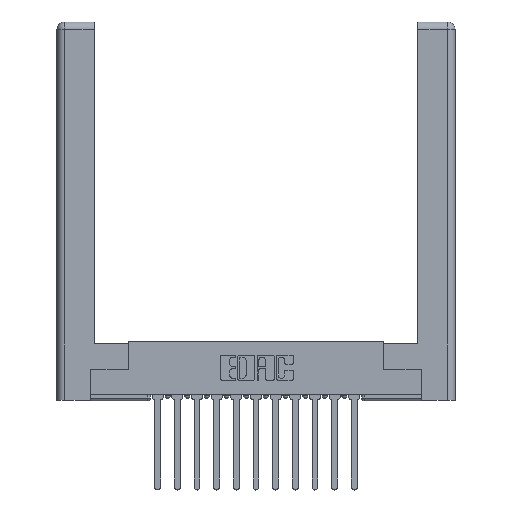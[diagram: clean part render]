
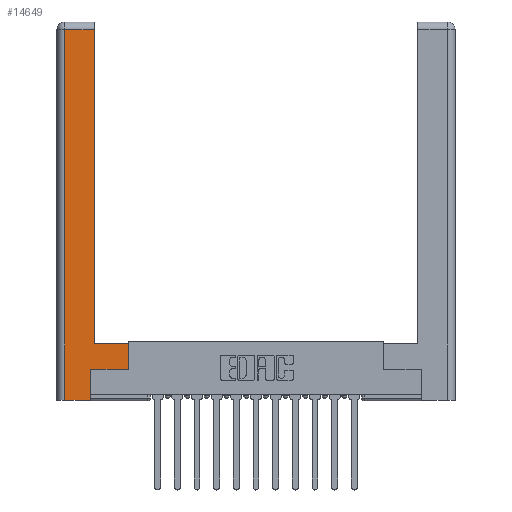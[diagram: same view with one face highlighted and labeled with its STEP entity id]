
A CAD part, top view. The second image highlights one B-rep face of the part: STEP entity #14649.
In plain terms, the highlighted planar face has unit normal (0, 0, 1).
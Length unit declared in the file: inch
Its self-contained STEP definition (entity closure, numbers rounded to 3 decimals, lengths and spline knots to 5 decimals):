
#219 = EDGE_CURVE ( 'NONE', #305, #6769, #8221, .T. ) ;
#305 = VERTEX_POINT ( 'NONE', #5192 ) ;
#957 = VERTEX_POINT ( 'NONE', #15986 ) ;
#1286 = DIRECTION ( 'NONE',  ( -1., 0., 0. ) ) ;
#1418 = DIRECTION ( 'NONE',  ( 0., 1., 0. ) ) ;
#1597 = CARTESIAN_POINT ( 'NONE',  ( 0.565, 0.45, 0. ) ) ;
#1611 = CARTESIAN_POINT ( 'NONE',  ( 0.565, 0.245, 0. ) ) ;
#1835 = VECTOR ( 'NONE', #6300, 39.37008 ) ;
#2227 = LINE ( 'NONE', #3310, #15348 ) ;
#2528 = VERTEX_POINT ( 'NONE', #7057 ) ;
#2570 = DIRECTION ( 'NONE',  ( 1., 0., 0. ) ) ;
#3310 = CARTESIAN_POINT ( 'NONE',  ( 0.265, 0.245, 0. ) ) ;
#3886 = CARTESIAN_POINT ( 'NONE',  ( 0.265, 0., 0. ) ) ;
#4019 = VECTOR ( 'NONE', #15083, 39.37008 ) ;
#4164 = EDGE_LOOP ( 'NONE', ( #5932, #5208, #7572, #6609, #14866, #4884, #8962, #14830 ) ) ;
#4169 = EDGE_CURVE ( 'NONE', #957, #11732, #12850, .T. ) ;
#4410 = LINE ( 'NONE', #11328, #4019 ) ;
#4884 = ORIENTED_EDGE ( 'NONE', *, *, #4169, .T. ) ;
#5192 = CARTESIAN_POINT ( 'NONE',  ( 0.0615, 0., 0. ) ) ;
#5208 = ORIENTED_EDGE ( 'NONE', *, *, #14543, .T. ) ;
#5555 = CARTESIAN_POINT ( 'NONE',  ( 0.0615, 2.94, 0. ) ) ;
#5618 = VECTOR ( 'NONE', #2570, 39.37008 ) ;
#5813 = DIRECTION ( 'NONE',  ( -1., 0., 0. ) ) ;
#5932 = ORIENTED_EDGE ( 'NONE', *, *, #9683, .T. ) ;
#6300 = DIRECTION ( 'NONE',  ( 1., 0., 0. ) ) ;
#6609 = ORIENTED_EDGE ( 'NONE', *, *, #219, .T. ) ;
#6634 = EDGE_CURVE ( 'NONE', #12723, #9093, #12505, .T. ) ;
#6769 = VERTEX_POINT ( 'NONE', #12047 ) ;
#7057 = CARTESIAN_POINT ( 'NONE',  ( 0.295, 2.94, 0. ) ) ;
#7165 = DIRECTION ( 'NONE',  ( 0., 0., -1. ) ) ;
#7258 = VECTOR ( 'NONE', #1418, 39.37008 ) ;
#7414 = FACE_OUTER_BOUND ( 'NONE', #4164, .T. ) ;
#7417 = DIRECTION ( 'NONE',  ( -1., 0., 0. ) ) ;
#7572 = ORIENTED_EDGE ( 'NONE', *, *, #14425, .T. ) ;
#7816 = LINE ( 'NONE', #13409, #12093 ) ;
#8221 = LINE ( 'NONE', #3886, #1835 ) ;
#8907 = CARTESIAN_POINT ( 'NONE',  ( 0.295, 0.45, 0. ) ) ;
#8962 = ORIENTED_EDGE ( 'NONE', *, *, #11346, .T. ) ;
#9093 = VERTEX_POINT ( 'NONE', #12573 ) ;
#9516 = CARTESIAN_POINT ( 'NONE',  ( 0.0615, 0., 0. ) ) ;
#9683 = EDGE_CURVE ( 'NONE', #9093, #2528, #4410, .T. ) ;
#9781 = CARTESIAN_POINT ( 'NONE',  ( 0., 0., 0. ) ) ;
#10582 = DIRECTION ( 'NONE',  ( 0., 1., 0. ) ) ;
#11236 = AXIS2_PLACEMENT_3D ( 'NONE', #9781, #7165, #7417 ) ;
#11328 = CARTESIAN_POINT ( 'NONE',  ( 0.295, 3., 0. ) ) ;
#11346 = EDGE_CURVE ( 'NONE', #11732, #12723, #14901, .T. ) ;
#11705 = VECTOR ( 'NONE', #1286, 39.37008 ) ;
#11732 = VERTEX_POINT ( 'NONE', #16099 ) ;
#12047 = CARTESIAN_POINT ( 'NONE',  ( 0.265, 0., 0. ) ) ;
#12093 = VECTOR ( 'NONE', #5813, 39.37008 ) ;
#12505 = LINE ( 'NONE', #8907, #11705 ) ;
#12573 = CARTESIAN_POINT ( 'NONE',  ( 0.295, 0.45, 0. ) ) ;
#12723 = VERTEX_POINT ( 'NONE', #1597 ) ;
#12850 = LINE ( 'NONE', #1611, #5618 ) ;
#12938 = EDGE_CURVE ( 'NONE', #6769, #957, #2227, .T. ) ;
#13409 = CARTESIAN_POINT ( 'NONE',  ( 0.0615, 2.94, 0. ) ) ;
#14296 = DIRECTION ( 'NONE',  ( 0., -1., 0. ) ) ;
#14371 = VERTEX_POINT ( 'NONE', #5555 ) ;
#14425 = EDGE_CURVE ( 'NONE', #14371, #305, #15486, .T. ) ;
#14497 = VECTOR ( 'NONE', #14296, 39.37008 ) ;
#14543 = EDGE_CURVE ( 'NONE', #2528, #14371, #7816, .T. ) ;
#14649 = ADVANCED_FACE ( 'NONE', ( #7414 ), #14665, .F. ) ;
#14665 = PLANE ( 'NONE',  #11236 ) ;
#14830 = ORIENTED_EDGE ( 'NONE', *, *, #6634, .T. ) ;
#14866 = ORIENTED_EDGE ( 'NONE', *, *, #12938, .T. ) ;
#14901 = LINE ( 'NONE', #15190, #7258 ) ;
#15083 = DIRECTION ( 'NONE',  ( 0., 1., 0. ) ) ;
#15190 = CARTESIAN_POINT ( 'NONE',  ( 0.565, 0.45, 0. ) ) ;
#15348 = VECTOR ( 'NONE', #10582, 39.37008 ) ;
#15486 = LINE ( 'NONE', #9516, #14497 ) ;
#15986 = CARTESIAN_POINT ( 'NONE',  ( 0.265, 0.245, 0. ) ) ;
#16099 = CARTESIAN_POINT ( 'NONE',  ( 0.565, 0.245, 0. ) ) ;
